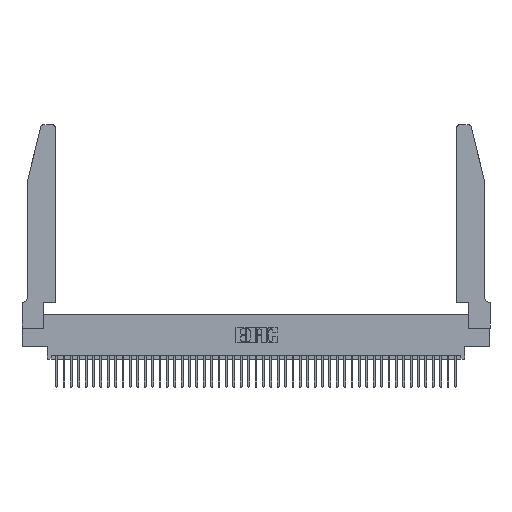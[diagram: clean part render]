
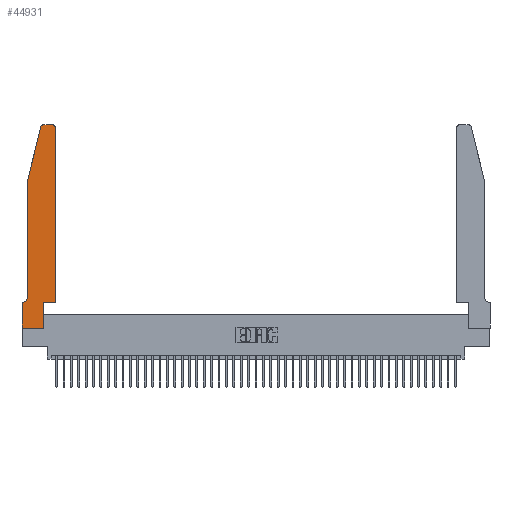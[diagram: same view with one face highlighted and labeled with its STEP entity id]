
A CAD part, top view. The second image highlights one B-rep face of the part: STEP entity #44931.
In plain terms, the highlighted planar face has unit normal (0, 0, 1).
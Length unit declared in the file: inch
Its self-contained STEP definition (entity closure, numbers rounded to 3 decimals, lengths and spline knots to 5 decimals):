
#101 = LINE ( 'NONE', #688, #37084 ) ;
#214 = VECTOR ( 'NONE', #2945, 39.37008 ) ;
#688 = CARTESIAN_POINT ( 'NONE',  ( 0.0755, 2., 0.37 ) ) ;
#944 = EDGE_CURVE ( 'NONE', #29747, #29710, #20416, .T. ) ;
#981 = ORIENTED_EDGE ( 'NONE', *, *, #33213, .T. ) ;
#1238 = VECTOR ( 'NONE', #35394, 39.37008 ) ;
#1364 = ORIENTED_EDGE ( 'NONE', *, *, #34173, .T. ) ;
#2648 = ORIENTED_EDGE ( 'NONE', *, *, #944, .T. ) ;
#2945 = DIRECTION ( 'NONE',  ( -1., 0., 0. ) ) ;
#3142 = DIRECTION ( 'NONE',  ( 1., 0., 0. ) ) ;
#3767 = EDGE_CURVE ( 'NONE', #21801, #7735, #101, .T. ) ;
#4453 = CARTESIAN_POINT ( 'NONE',  ( 0., 0., 0.37 ) ) ;
#4485 = DIRECTION ( 'NONE',  ( -0.239, -0.971, 0. ) ) ;
#5031 = CARTESIAN_POINT ( 'NONE',  ( 0.0055, 0.42, 0.37 ) ) ;
#6024 = ORIENTED_EDGE ( 'NONE', *, *, #40425, .T. ) ;
#6439 = AXIS2_PLACEMENT_3D ( 'NONE', #45964, #24603, #3142 ) ;
#7055 = CIRCLE ( 'NONE', #6439, 0.03 ) ;
#7090 = ORIENTED_EDGE ( 'NONE', *, *, #19630, .T. ) ;
#7392 = CARTESIAN_POINT ( 'NONE',  ( 0., 0.35, 0.37 ) ) ;
#7735 = VERTEX_POINT ( 'NONE', #8083 ) ;
#8083 = CARTESIAN_POINT ( 'NONE',  ( 0.0755, 2., 0.37 ) ) ;
#8488 = CIRCLE ( 'NONE', #37498, 0.07 ) ;
#8640 = DIRECTION ( 'NONE',  ( -1., 0., 0. ) ) ;
#9244 = CARTESIAN_POINT ( 'NONE',  ( 0., 0., 0.37 ) ) ;
#9247 = AXIS2_PLACEMENT_3D ( 'NONE', #36791, #11982, #36948 ) ;
#9783 = VERTEX_POINT ( 'NONE', #37459 ) ;
#11982 = DIRECTION ( 'NONE',  ( 0., 0., 1. ) ) ;
#11987 = EDGE_CURVE ( 'NONE', #43733, #18761, #36562, .T. ) ;
#12164 = EDGE_CURVE ( 'NONE', #24744, #9783, #32109, .T. ) ;
#12899 = DIRECTION ( 'NONE',  ( 0., 0., 1. ) ) ;
#14387 = VECTOR ( 'NONE', #29152, 39.37008 ) ;
#15603 = CARTESIAN_POINT ( 'NONE',  ( 0., 0., 0.37 ) ) ;
#16811 = FACE_OUTER_BOUND ( 'NONE', #44387, .T. ) ;
#17146 = CARTESIAN_POINT ( 'NONE',  ( 0.25487, 2.72718, 0.37 ) ) ;
#17552 = VECTOR ( 'NONE', #42154, 39.37008 ) ;
#18151 = ORIENTED_EDGE ( 'NONE', *, *, #3767, .T. ) ;
#18761 = VERTEX_POINT ( 'NONE', #33284 ) ;
#18845 = DIRECTION ( 'NONE',  ( 1., 0., 0. ) ) ;
#19630 = EDGE_CURVE ( 'NONE', #38571, #23202, #39152, .T. ) ;
#20329 = VECTOR ( 'NONE', #21713, 39.37008 ) ;
#20416 = LINE ( 'NONE', #24402, #214 ) ;
#20605 = CARTESIAN_POINT ( 'NONE',  ( 0.0055, 0.35, 0.37 ) ) ;
#20932 = CARTESIAN_POINT ( 'NONE',  ( 0.4205, 2.75, 0.37 ) ) ;
#21325 = ORIENTED_EDGE ( 'NONE', *, *, #35575, .T. ) ;
#21713 = DIRECTION ( 'NONE',  ( 0., 1., 0. ) ) ;
#21801 = VERTEX_POINT ( 'NONE', #17146 ) ;
#23202 = VERTEX_POINT ( 'NONE', #15603 ) ;
#24033 = AXIS2_PLACEMENT_3D ( 'NONE', #34350, #12899, #37883 ) ;
#24402 = CARTESIAN_POINT ( 'NONE',  ( 0.2605, 2.75, 0.37 ) ) ;
#24603 = DIRECTION ( 'NONE',  ( 0., 0., 1. ) ) ;
#24744 = VERTEX_POINT ( 'NONE', #38260 ) ;
#25529 = CARTESIAN_POINT ( 'NONE',  ( 0.0755, 2., 0.37 ) ) ;
#25838 = LINE ( 'NONE', #45702, #34242 ) ;
#26192 = PLANE ( 'NONE',  #9247 ) ;
#26388 = CIRCLE ( 'NONE', #24033, 0.03 ) ;
#26641 = EDGE_CURVE ( 'NONE', #7735, #28994, #34560, .T. ) ;
#27095 = VERTEX_POINT ( 'NONE', #20605 ) ;
#27971 = DIRECTION ( 'NONE',  ( 1., 0., 0. ) ) ;
#28272 = ORIENTED_EDGE ( 'NONE', *, *, #11987, .T. ) ;
#28994 = VERTEX_POINT ( 'NONE', #44709 ) ;
#29152 = DIRECTION ( 'NONE',  ( 0., -1., 0. ) ) ;
#29710 = VERTEX_POINT ( 'NONE', #45426 ) ;
#29747 = VERTEX_POINT ( 'NONE', #20932 ) ;
#29871 = LINE ( 'NONE', #31801, #1238 ) ;
#30101 = DIRECTION ( 'NONE',  ( 0., 0., -1. ) ) ;
#30825 = VECTOR ( 'NONE', #37837, 39.37008 ) ;
#31349 = ORIENTED_EDGE ( 'NONE', *, *, #26641, .T. ) ;
#31801 = CARTESIAN_POINT ( 'NONE',  ( 0.0755, 0.35, 0.37 ) ) ;
#32109 = LINE ( 'NONE', #43072, #20329 ) ;
#33213 = EDGE_CURVE ( 'NONE', #28994, #27095, #8488, .T. ) ;
#33284 = CARTESIAN_POINT ( 'NONE',  ( 0.4505, 2.72, 0.37 ) ) ;
#33334 = CARTESIAN_POINT ( 'NONE',  ( 0.4505, 0.35, 0.37 ) ) ;
#34173 = EDGE_CURVE ( 'NONE', #9783, #43733, #25838, .T. ) ;
#34242 = VECTOR ( 'NONE', #27971, 39.37008 ) ;
#34350 = CARTESIAN_POINT ( 'NONE',  ( 0.284, 2.72, 0.37 ) ) ;
#34545 = ORIENTED_EDGE ( 'NONE', *, *, #37257, .T. ) ;
#34560 = LINE ( 'NONE', #25529, #14387 ) ;
#35367 = VECTOR ( 'NONE', #18845, 39.37008 ) ;
#35394 = DIRECTION ( 'NONE',  ( -1., 0., 0. ) ) ;
#35575 = EDGE_CURVE ( 'NONE', #27095, #38571, #29871, .T. ) ;
#36562 = LINE ( 'NONE', #38562, #17552 ) ;
#36791 = CARTESIAN_POINT ( 'NONE',  ( 0., 0.35, 0.37 ) ) ;
#36948 = DIRECTION ( 'NONE',  ( 1., 0., 0. ) ) ;
#37048 = EDGE_CURVE ( 'NONE', #23202, #24744, #44805, .T. ) ;
#37084 = VECTOR ( 'NONE', #4485, 39.37008 ) ;
#37257 = EDGE_CURVE ( 'NONE', #29710, #21801, #26388, .T. ) ;
#37459 = CARTESIAN_POINT ( 'NONE',  ( 0.2865, 0.35, 0.37 ) ) ;
#37498 = AXIS2_PLACEMENT_3D ( 'NONE', #5031, #30101, #8640 ) ;
#37837 = DIRECTION ( 'NONE',  ( 0., -1., 0. ) ) ;
#37883 = DIRECTION ( 'NONE',  ( 1., 0., 0. ) ) ;
#38260 = CARTESIAN_POINT ( 'NONE',  ( 0.2865, 0., 0.37 ) ) ;
#38562 = CARTESIAN_POINT ( 'NONE',  ( 0.4505, 0.35, 0.37 ) ) ;
#38571 = VERTEX_POINT ( 'NONE', #7392 ) ;
#39152 = LINE ( 'NONE', #9244, #30825 ) ;
#40425 = EDGE_CURVE ( 'NONE', #18761, #29747, #7055, .T. ) ;
#42154 = DIRECTION ( 'NONE',  ( 0., 1., 0. ) ) ;
#43072 = CARTESIAN_POINT ( 'NONE',  ( 0.2865, 0.35, 0.37 ) ) ;
#43733 = VERTEX_POINT ( 'NONE', #33334 ) ;
#44330 = ORIENTED_EDGE ( 'NONE', *, *, #12164, .T. ) ;
#44387 = EDGE_LOOP ( 'NONE', ( #2648, #34545, #18151, #31349, #981, #21325, #7090, #44598, #44330, #1364, #28272, #6024 ) ) ;
#44598 = ORIENTED_EDGE ( 'NONE', *, *, #37048, .T. ) ;
#44709 = CARTESIAN_POINT ( 'NONE',  ( 0.0755, 0.42, 0.37 ) ) ;
#44805 = LINE ( 'NONE', #4453, #35367 ) ;
#44931 = ADVANCED_FACE ( 'NONE', ( #16811 ), #26192, .T. ) ;
#45426 = CARTESIAN_POINT ( 'NONE',  ( 0.284, 2.75, 0.37 ) ) ;
#45702 = CARTESIAN_POINT ( 'NONE',  ( 0.4505, 0.35, 0.37 ) ) ;
#45964 = CARTESIAN_POINT ( 'NONE',  ( 0.4205, 2.72, 0.37 ) ) ;
